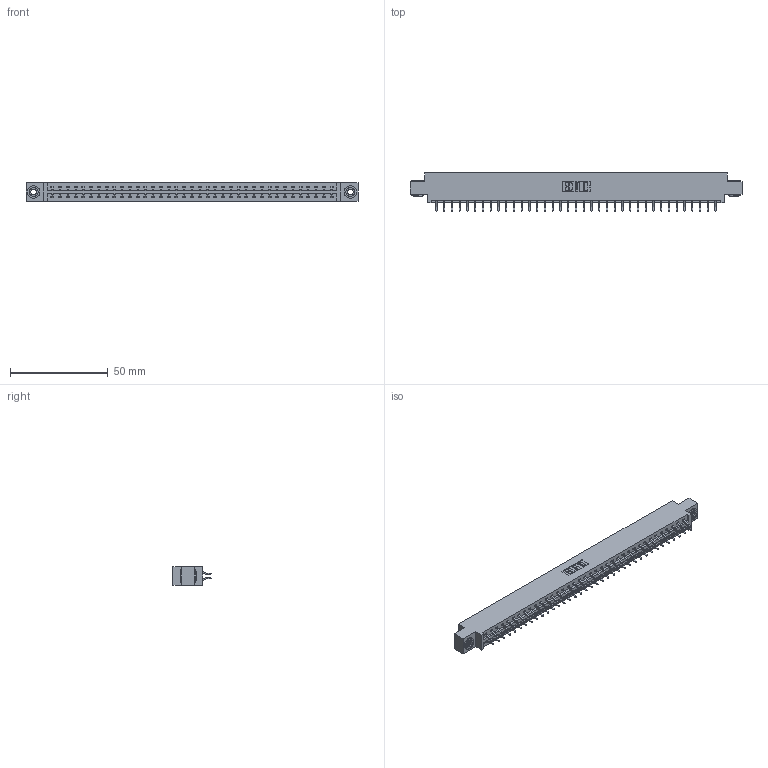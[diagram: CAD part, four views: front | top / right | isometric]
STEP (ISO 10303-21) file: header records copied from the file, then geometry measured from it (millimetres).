
FILE_DESCRIPTION (( 'STEP AP203' ), '1' );
FILE_NAME ('337-074-556-803.STEP', '2019-10-15T12:44:37', ( '' ), ( '' ), 'SwSTEP 2.0', 'SolidWorks 2016', '' );
FILE_SCHEMA (( 'CONFIG_CONTROL_DESIGN' ));
Length unit declared in the file: inch
Products named in the file (4): 345-250-002_345-250-002-102; 345-292-001_556 Tail; 337 Part_0.170 Offset - 0.156 Dia-TH; 337-074-556-803
Assembly tree (77 placements, depth 2):
  337-074-556-803
    337 Part_0.170 Offset - 0.156 Dia-TH
    345-292-001_556 Tail  x74
    345-250-002_345-250-002-102  x2
Bounding box: 169.62 x 19.57 x 9.4 mm (x, y, z)
Volume: 17708.4 mm3; surface area: 20225 mm2
Topology: 77 solids, 77 shells, 4596 faces, 13645 edges, 8994 vertices
Faces by surface type: plane 3192, cylinder 1396, cone 8
Entity records: 30336 total; most frequent: CARTESIAN_POINT 5105, ORIENTED_EDGE 5022, DIRECTION 4373, EDGE_CURVE 2511, VECTOR 2351, LINE 2351, VERTEX_POINT 1670, AXIS2_PLACEMENT_3D 1011
